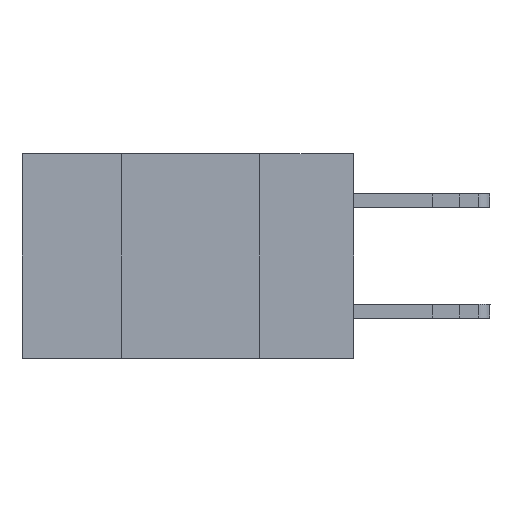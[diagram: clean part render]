
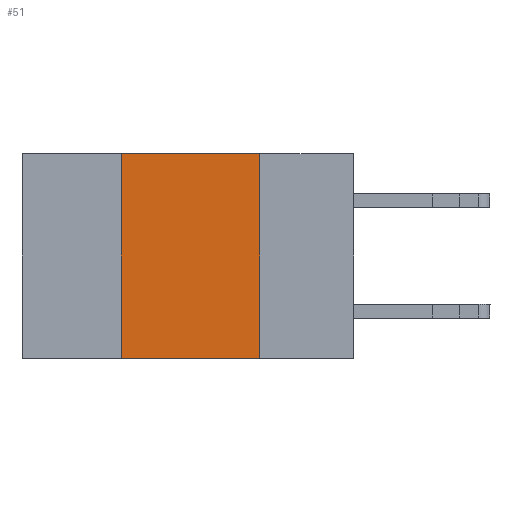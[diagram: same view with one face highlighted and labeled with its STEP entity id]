
A CAD part, left-side view. The second image highlights one B-rep face of the part: STEP entity #51.
In plain terms, the highlighted planar face has unit normal (-1, 0, 0).
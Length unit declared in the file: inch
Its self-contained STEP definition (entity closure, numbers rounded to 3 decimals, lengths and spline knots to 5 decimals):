
#51 = ADVANCED_FACE ( 'NONE', ( #14303 ), #4714, .F. ) ;
#154 = VECTOR ( 'NONE', #15349, 39.37008 ) ;
#564 = VECTOR ( 'NONE', #11292, 39.37008 ) ;
#805 = CARTESIAN_POINT ( 'NONE',  ( 0., 0.42, -0.37 ) ) ;
#1275 = EDGE_LOOP ( 'NONE', ( #16890, #3276, #14274, #17975 ) ) ;
#2003 = CARTESIAN_POINT ( 'NONE',  ( 0., 0.42, 0. ) ) ;
#2750 = VERTEX_POINT ( 'NONE', #12527 ) ;
#3112 = VERTEX_POINT ( 'NONE', #12235 ) ;
#3276 = ORIENTED_EDGE ( 'NONE', *, *, #16925, .F. ) ;
#4175 = LINE ( 'NONE', #15149, #8650 ) ;
#4526 = VECTOR ( 'NONE', #4840, 39.37008 ) ;
#4714 = PLANE ( 'NONE',  #13103 ) ;
#4840 = DIRECTION ( 'NONE',  ( 0., 0., 1. ) ) ;
#7109 = LINE ( 'NONE', #8473, #564 ) ;
#7353 = DIRECTION ( 'NONE',  ( 1., 0., 0. ) ) ;
#8473 = CARTESIAN_POINT ( 'NONE',  ( 0., 0.6, -0.37 ) ) ;
#8650 = VECTOR ( 'NONE', #9654, 39.37008 ) ;
#8721 = CARTESIAN_POINT ( 'NONE',  ( 0., 0.6, 0. ) ) ;
#8815 = DIRECTION ( 'NONE',  ( 0., 0., -1. ) ) ;
#9654 = DIRECTION ( 'NONE',  ( 0., 0., -1. ) ) ;
#9673 = CARTESIAN_POINT ( 'NONE',  ( 0., 0.17, 0. ) ) ;
#9760 = CARTESIAN_POINT ( 'NONE',  ( 0., 0.6, 0. ) ) ;
#10072 = EDGE_CURVE ( 'NONE', #17266, #2750, #7109, .T. ) ;
#11207 = VERTEX_POINT ( 'NONE', #9673 ) ;
#11292 = DIRECTION ( 'NONE',  ( 0., -1., 0. ) ) ;
#12235 = CARTESIAN_POINT ( 'NONE',  ( 0., 0.42, 0. ) ) ;
#12527 = CARTESIAN_POINT ( 'NONE',  ( 0., 0.17, -0.37 ) ) ;
#13103 = AXIS2_PLACEMENT_3D ( 'NONE', #8721, #7353, #8815 ) ;
#14247 = EDGE_CURVE ( 'NONE', #11207, #2750, #4175, .T. ) ;
#14274 = ORIENTED_EDGE ( 'NONE', *, *, #18049, .F. ) ;
#14303 = FACE_OUTER_BOUND ( 'NONE', #1275, .T. ) ;
#14961 = LINE ( 'NONE', #2003, #4526 ) ;
#15149 = CARTESIAN_POINT ( 'NONE',  ( 0., 0.17, 0. ) ) ;
#15349 = DIRECTION ( 'NONE',  ( 0., -1., 0. ) ) ;
#16724 = LINE ( 'NONE', #9760, #154 ) ;
#16890 = ORIENTED_EDGE ( 'NONE', *, *, #14247, .F. ) ;
#16925 = EDGE_CURVE ( 'NONE', #3112, #11207, #16724, .T. ) ;
#17266 = VERTEX_POINT ( 'NONE', #805 ) ;
#17975 = ORIENTED_EDGE ( 'NONE', *, *, #10072, .T. ) ;
#18049 = EDGE_CURVE ( 'NONE', #17266, #3112, #14961, .T. ) ;
